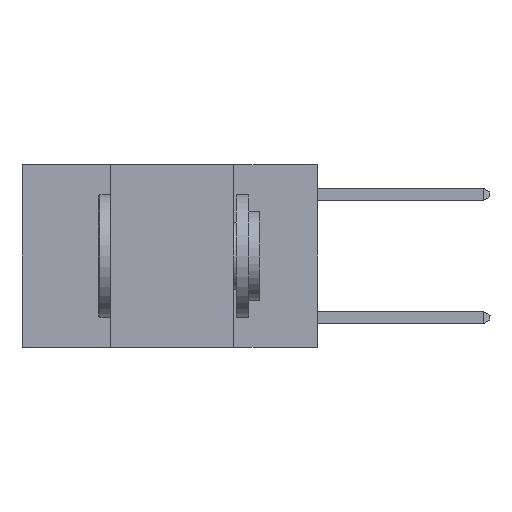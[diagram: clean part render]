
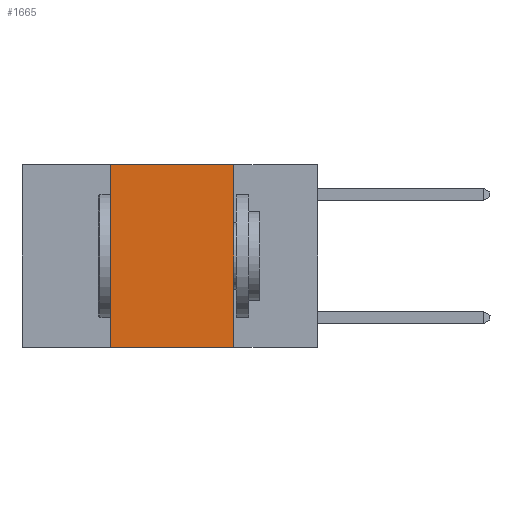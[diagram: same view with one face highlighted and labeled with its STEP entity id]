
A CAD part, left-side view. The second image highlights one B-rep face of the part: STEP entity #1665.
In plain terms, the highlighted planar face has unit normal (-1, 0, 0).
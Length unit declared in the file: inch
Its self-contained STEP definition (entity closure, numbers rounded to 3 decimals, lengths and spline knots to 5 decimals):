
#33 = EDGE_CURVE ( 'NONE', #6372, #12000, #6681, .T. ) ;
#553 = ORIENTED_EDGE ( 'NONE', *, *, #11734, .F. ) ;
#1013 = DIRECTION ( 'NONE',  ( 0., 0., -1. ) ) ;
#1183 = DIRECTION ( 'NONE',  ( 1., 0., 0. ) ) ;
#1543 = PLANE ( 'NONE',  #9015 ) ;
#1665 = ADVANCED_FACE ( 'NONE', ( #12710 ), #1543, .F. ) ;
#2067 = VERTEX_POINT ( 'NONE', #14512 ) ;
#2140 = ORIENTED_EDGE ( 'NONE', *, *, #14984, .T. ) ;
#2226 = LINE ( 'NONE', #14550, #8171 ) ;
#2389 = CARTESIAN_POINT ( 'NONE',  ( 0., 0.42, 0. ) ) ;
#3596 = VERTEX_POINT ( 'NONE', #5458 ) ;
#3934 = ORIENTED_EDGE ( 'NONE', *, *, #33, .F. ) ;
#3977 = CARTESIAN_POINT ( 'NONE',  ( 0., 0.17, 0. ) ) ;
#4254 = VECTOR ( 'NONE', #4935, 39.37008 ) ;
#4589 = CARTESIAN_POINT ( 'NONE',  ( 0., 0.6, 0. ) ) ;
#4935 = DIRECTION ( 'NONE',  ( 0., 0., 1. ) ) ;
#4996 = DIRECTION ( 'NONE',  ( 0., -1., 0. ) ) ;
#5101 = VECTOR ( 'NONE', #12306, 39.37008 ) ;
#5458 = CARTESIAN_POINT ( 'NONE',  ( 0., 0.17, -0.37 ) ) ;
#5719 = DIRECTION ( 'NONE',  ( 0., -1., 0. ) ) ;
#5836 = EDGE_LOOP ( 'NONE', ( #553, #3934, #8083, #2140 ) ) ;
#6031 = CARTESIAN_POINT ( 'NONE',  ( 0., 0.17, 0. ) ) ;
#6372 = VERTEX_POINT ( 'NONE', #9526 ) ;
#6681 = LINE ( 'NONE', #14094, #9992 ) ;
#7619 = LINE ( 'NONE', #2389, #4254 ) ;
#8083 = ORIENTED_EDGE ( 'NONE', *, *, #13863, .F. ) ;
#8171 = VECTOR ( 'NONE', #5719, 39.37008 ) ;
#9015 = AXIS2_PLACEMENT_3D ( 'NONE', #4589, #1183, #1013 ) ;
#9526 = CARTESIAN_POINT ( 'NONE',  ( 0., 0.42, 0. ) ) ;
#9992 = VECTOR ( 'NONE', #4996, 39.37008 ) ;
#11734 = EDGE_CURVE ( 'NONE', #12000, #3596, #12190, .T. ) ;
#12000 = VERTEX_POINT ( 'NONE', #3977 ) ;
#12190 = LINE ( 'NONE', #6031, #5101 ) ;
#12306 = DIRECTION ( 'NONE',  ( 0., 0., -1. ) ) ;
#12710 = FACE_OUTER_BOUND ( 'NONE', #5836, .T. ) ;
#13863 = EDGE_CURVE ( 'NONE', #2067, #6372, #7619, .T. ) ;
#14094 = CARTESIAN_POINT ( 'NONE',  ( 0., 0.6, 0. ) ) ;
#14512 = CARTESIAN_POINT ( 'NONE',  ( 0., 0.42, -0.37 ) ) ;
#14550 = CARTESIAN_POINT ( 'NONE',  ( 0., 0.6, -0.37 ) ) ;
#14984 = EDGE_CURVE ( 'NONE', #2067, #3596, #2226, .T. ) ;
